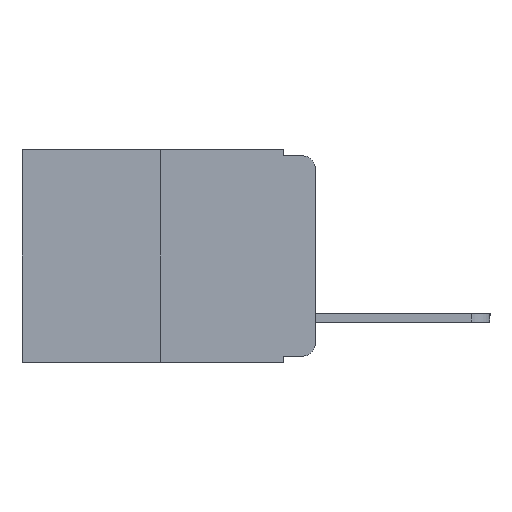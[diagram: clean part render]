
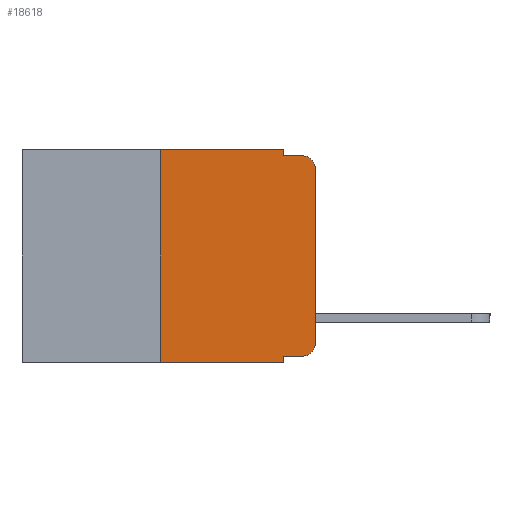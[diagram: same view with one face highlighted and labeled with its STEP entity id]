
A CAD part, left-side view. The second image highlights one B-rep face of the part: STEP entity #18618.
In plain terms, the highlighted planar face has unit normal (-1, 0, 0).
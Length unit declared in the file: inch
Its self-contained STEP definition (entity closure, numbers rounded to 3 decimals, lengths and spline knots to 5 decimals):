
#89 = VERTEX_POINT ( 'NONE', #1777 ) ;
#171 = VECTOR ( 'NONE', #8362, 39.37008 ) ;
#450 = VECTOR ( 'NONE', #16243, 39.37008 ) ;
#452 = DIRECTION ( 'NONE',  ( 0., 0., -1. ) ) ;
#640 = CARTESIAN_POINT ( 'NONE',  ( 0., 0.25, 0. ) ) ;
#958 = EDGE_CURVE ( 'NONE', #12608, #5163, #18054, .T. ) ;
#959 = EDGE_CURVE ( 'NONE', #5163, #8578, #10864, .T. ) ;
#1000 = EDGE_CURVE ( 'NONE', #4320, #8578, #6597, .T. ) ;
#1128 = EDGE_CURVE ( 'NONE', #7539, #4320, #12794, .T. ) ;
#1162 = EDGE_CURVE ( 'NONE', #7842, #3371, #12381, .T. ) ;
#1278 = ORIENTED_EDGE ( 'NONE', *, *, #1455, .T. ) ;
#1294 = EDGE_CURVE ( 'NONE', #12887, #89, #14266, .T. ) ;
#1455 = EDGE_CURVE ( 'NONE', #12887, #19004, #12991, .T. ) ;
#1459 = EDGE_CURVE ( 'NONE', #19004, #12608, #9151, .T. ) ;
#1777 = CARTESIAN_POINT ( 'NONE',  ( 0., 0.051, -0.343 ) ) ;
#2099 = PLANE ( 'NONE',  #16049 ) ;
#2330 = VECTOR ( 'NONE', #7181, 39.37008 ) ;
#2915 = CARTESIAN_POINT ( 'NONE',  ( 0., 0.25, 0. ) ) ;
#2994 = CARTESIAN_POINT ( 'NONE',  ( 0., 0.051, -0.01 ) ) ;
#3371 = VERTEX_POINT ( 'NONE', #2915 ) ;
#3464 = CARTESIAN_POINT ( 'NONE',  ( 0., 0.02, -0.01 ) ) ;
#3762 = EDGE_LOOP ( 'NONE', ( #6826, #14641, #15057, #4550, #16335, #5031, #13184, #16743, #1278, #13608 ) ) ;
#3834 = DIRECTION ( 'NONE',  ( 0., -1., 0. ) ) ;
#4027 = DIRECTION ( 'NONE',  ( 0., 0., -1. ) ) ;
#4320 = VERTEX_POINT ( 'NONE', #2994 ) ;
#4550 = ORIENTED_EDGE ( 'NONE', *, *, #1128, .F. ) ;
#4972 = LINE ( 'NONE', #6055, #12717 ) ;
#5031 = ORIENTED_EDGE ( 'NONE', *, *, #1162, .F. ) ;
#5096 = DIRECTION ( 'NONE',  ( 0., -1., 0. ) ) ;
#5163 = VERTEX_POINT ( 'NONE', #8705 ) ;
#5371 = CARTESIAN_POINT ( 'NONE',  ( 0., 0.02, -0.313 ) ) ;
#5443 = VECTOR ( 'NONE', #5096, 39.37008 ) ;
#6055 = CARTESIAN_POINT ( 'NONE',  ( 0., 0.473, 0. ) ) ;
#6338 = VECTOR ( 'NONE', #8754, 39.37008 ) ;
#6585 = CARTESIAN_POINT ( 'NONE',  ( 0., 0.02, -0.333 ) ) ;
#6597 = LINE ( 'NONE', #14153, #9912 ) ;
#6667 = CARTESIAN_POINT ( 'NONE',  ( 0., 0.473, -0.343 ) ) ;
#6826 = ORIENTED_EDGE ( 'NONE', *, *, #958, .T. ) ;
#6974 = FACE_OUTER_BOUND ( 'NONE', #3762, .T. ) ;
#7181 = DIRECTION ( 'NONE',  ( 0., 0., 1. ) ) ;
#7539 = VERTEX_POINT ( 'NONE', #13696 ) ;
#7704 = DIRECTION ( 'NONE',  ( 0., -1., 0. ) ) ;
#7842 = VERTEX_POINT ( 'NONE', #10706 ) ;
#8362 = DIRECTION ( 'NONE',  ( 0., 0., -1. ) ) ;
#8502 = CARTESIAN_POINT ( 'NONE',  ( 0., 0.051, 0. ) ) ;
#8578 = VERTEX_POINT ( 'NONE', #3464 ) ;
#8705 = CARTESIAN_POINT ( 'NONE',  ( 0., 0., -0.03 ) ) ;
#8754 = DIRECTION ( 'NONE',  ( 0., 0., -1. ) ) ;
#9151 = CIRCLE ( 'NONE', #12830, 0.02 ) ;
#9795 = LINE ( 'NONE', #6667, #5443 ) ;
#9912 = VECTOR ( 'NONE', #3834, 39.37008 ) ;
#10225 = DIRECTION ( 'NONE',  ( 1., 0., 0. ) ) ;
#10706 = CARTESIAN_POINT ( 'NONE',  ( 0., 0.25, -0.343 ) ) ;
#10728 = CARTESIAN_POINT ( 'NONE',  ( 0., 0., -0.313 ) ) ;
#10777 = EDGE_CURVE ( 'NONE', #7842, #89, #9795, .T. ) ;
#10864 = CIRCLE ( 'NONE', #12263, 0.02 ) ;
#11829 = CARTESIAN_POINT ( 'NONE',  ( 0., 0.051, 0. ) ) ;
#12263 = AXIS2_PLACEMENT_3D ( 'NONE', #12857, #12895, #4027 ) ;
#12381 = LINE ( 'NONE', #640, #15510 ) ;
#12608 = VERTEX_POINT ( 'NONE', #10728 ) ;
#12717 = VECTOR ( 'NONE', #7704, 39.37008 ) ;
#12794 = LINE ( 'NONE', #8502, #171 ) ;
#12830 = AXIS2_PLACEMENT_3D ( 'NONE', #5371, #17191, #15315 ) ;
#12857 = CARTESIAN_POINT ( 'NONE',  ( 0., 0.02, -0.03 ) ) ;
#12887 = VERTEX_POINT ( 'NONE', #17743 ) ;
#12895 = DIRECTION ( 'NONE',  ( -1., 0., 0. ) ) ;
#12991 = LINE ( 'NONE', #14677, #450 ) ;
#13184 = ORIENTED_EDGE ( 'NONE', *, *, #10777, .T. ) ;
#13608 = ORIENTED_EDGE ( 'NONE', *, *, #1459, .T. ) ;
#13696 = CARTESIAN_POINT ( 'NONE',  ( 0., 0.051, 0. ) ) ;
#14153 = CARTESIAN_POINT ( 'NONE',  ( 0., 0.051, -0.01 ) ) ;
#14214 = DIRECTION ( 'NONE',  ( 0., 0., 1. ) ) ;
#14266 = LINE ( 'NONE', #11829, #6338 ) ;
#14315 = CARTESIAN_POINT ( 'NONE',  ( 0., 0.473, 0. ) ) ;
#14325 = CARTESIAN_POINT ( 'NONE',  ( 0., 0., 0. ) ) ;
#14641 = ORIENTED_EDGE ( 'NONE', *, *, #959, .T. ) ;
#14677 = CARTESIAN_POINT ( 'NONE',  ( 0., 0.051, -0.333 ) ) ;
#15057 = ORIENTED_EDGE ( 'NONE', *, *, #1000, .F. ) ;
#15315 = DIRECTION ( 'NONE',  ( 0., 0., -1. ) ) ;
#15510 = VECTOR ( 'NONE', #14214, 39.37008 ) ;
#16049 = AXIS2_PLACEMENT_3D ( 'NONE', #14315, #10225, #452 ) ;
#16243 = DIRECTION ( 'NONE',  ( 0., -1., 0. ) ) ;
#16335 = ORIENTED_EDGE ( 'NONE', *, *, #17705, .F. ) ;
#16743 = ORIENTED_EDGE ( 'NONE', *, *, #1294, .F. ) ;
#17191 = DIRECTION ( 'NONE',  ( -1., 0., 0. ) ) ;
#17705 = EDGE_CURVE ( 'NONE', #3371, #7539, #4972, .T. ) ;
#17743 = CARTESIAN_POINT ( 'NONE',  ( 0., 0.051, -0.333 ) ) ;
#18054 = LINE ( 'NONE', #14325, #2330 ) ;
#18618 = ADVANCED_FACE ( 'NONE', ( #6974 ), #2099, .F. ) ;
#19004 = VERTEX_POINT ( 'NONE', #6585 ) ;
